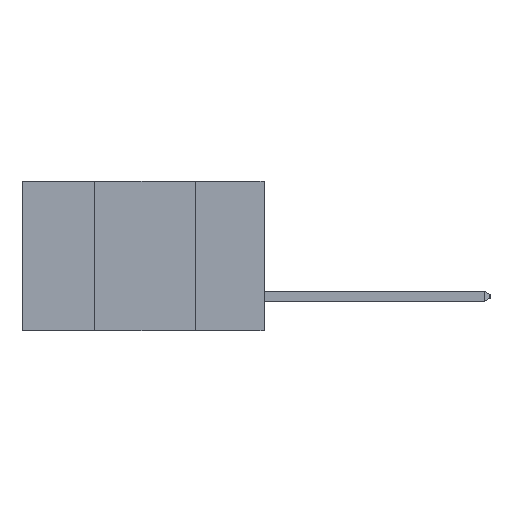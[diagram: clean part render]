
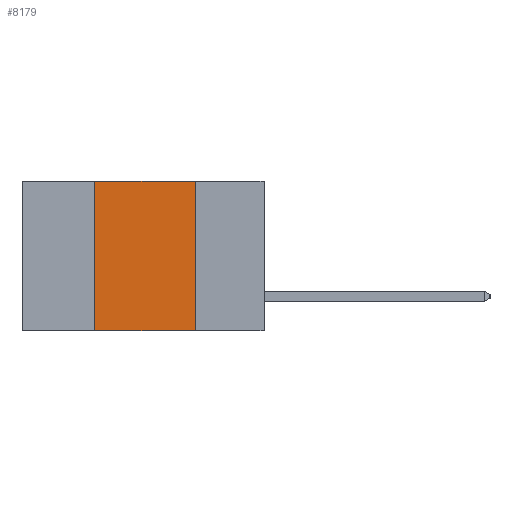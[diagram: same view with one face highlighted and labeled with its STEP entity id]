
A CAD part, left-side view. The second image highlights one B-rep face of the part: STEP entity #8179.
In plain terms, the highlighted planar face has unit normal (-1, 0, 0).
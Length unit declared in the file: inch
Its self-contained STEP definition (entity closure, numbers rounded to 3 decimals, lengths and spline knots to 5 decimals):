
#54 = ORIENTED_EDGE ( 'NONE', *, *, #4067, .F. ) ;
#656 = EDGE_LOOP ( 'NONE', ( #3995, #54, #10263, #1364 ) ) ;
#931 = VERTEX_POINT ( 'NONE', #6110 ) ;
#1364 = ORIENTED_EDGE ( 'NONE', *, *, #5217, .T. ) ;
#1379 = AXIS2_PLACEMENT_3D ( 'NONE', #9594, #9261, #9206 ) ;
#1904 = LINE ( 'NONE', #7012, #5973 ) ;
#2960 = LINE ( 'NONE', #5748, #5002 ) ;
#2989 = VERTEX_POINT ( 'NONE', #5618 ) ;
#3473 = EDGE_CURVE ( 'NONE', #931, #4764, #4457, .T. ) ;
#3995 = ORIENTED_EDGE ( 'NONE', *, *, #3473, .F. ) ;
#4067 = EDGE_CURVE ( 'NONE', #2989, #931, #1904, .T. ) ;
#4457 = LINE ( 'NONE', #10538, #6202 ) ;
#4561 = DIRECTION ( 'NONE',  ( 0., 0., 1. ) ) ;
#4657 = EDGE_CURVE ( 'NONE', #9705, #2989, #8509, .T. ) ;
#4746 = CARTESIAN_POINT ( 'NONE',  ( 0., 0.42, -0.37 ) ) ;
#4764 = VERTEX_POINT ( 'NONE', #7983 ) ;
#5002 = VECTOR ( 'NONE', #8520, 39.37008 ) ;
#5217 = EDGE_CURVE ( 'NONE', #9705, #4764, #2960, .T. ) ;
#5618 = CARTESIAN_POINT ( 'NONE',  ( 0., 0.42, 0. ) ) ;
#5715 = CARTESIAN_POINT ( 'NONE',  ( 0., 0.42, -0.37 ) ) ;
#5748 = CARTESIAN_POINT ( 'NONE',  ( 0., 0.6, -0.37 ) ) ;
#5973 = VECTOR ( 'NONE', #7496, 39.37008 ) ;
#6110 = CARTESIAN_POINT ( 'NONE',  ( 0., 0.17, 0. ) ) ;
#6202 = VECTOR ( 'NONE', #10577, 39.37008 ) ;
#6362 = VECTOR ( 'NONE', #4561, 39.37008 ) ;
#7012 = CARTESIAN_POINT ( 'NONE',  ( 0., 0.6, 0. ) ) ;
#7496 = DIRECTION ( 'NONE',  ( 0., -1., 0. ) ) ;
#7983 = CARTESIAN_POINT ( 'NONE',  ( 0., 0.17, -0.37 ) ) ;
#8179 = ADVANCED_FACE ( 'NONE', ( #10714 ), #9562, .F. ) ;
#8509 = LINE ( 'NONE', #4746, #6362 ) ;
#8520 = DIRECTION ( 'NONE',  ( 0., -1., 0. ) ) ;
#9206 = DIRECTION ( 'NONE',  ( 0., 0., -1. ) ) ;
#9261 = DIRECTION ( 'NONE',  ( 1., 0., 0. ) ) ;
#9562 = PLANE ( 'NONE',  #1379 ) ;
#9594 = CARTESIAN_POINT ( 'NONE',  ( 0., 0.6, 0. ) ) ;
#9705 = VERTEX_POINT ( 'NONE', #5715 ) ;
#10263 = ORIENTED_EDGE ( 'NONE', *, *, #4657, .F. ) ;
#10538 = CARTESIAN_POINT ( 'NONE',  ( 0., 0.17, -0.37 ) ) ;
#10577 = DIRECTION ( 'NONE',  ( 0., 0., -1. ) ) ;
#10714 = FACE_OUTER_BOUND ( 'NONE', #656, .T. ) ;
